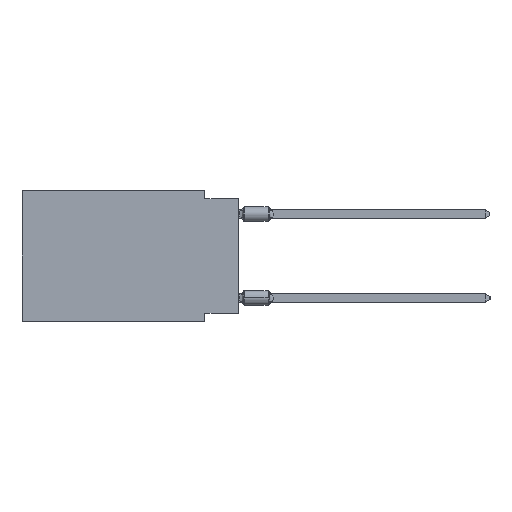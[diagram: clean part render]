
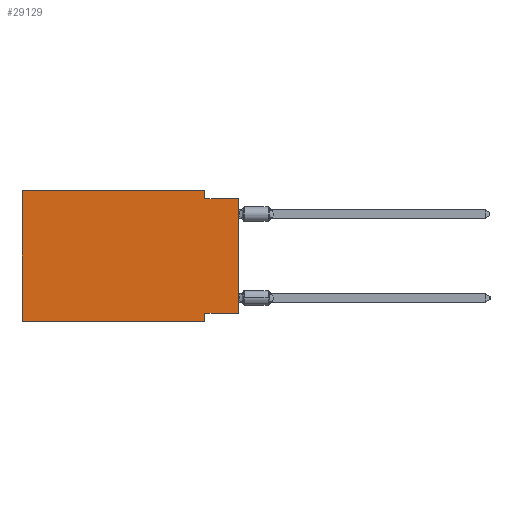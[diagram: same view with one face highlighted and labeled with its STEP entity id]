
A CAD part, left-side view. The second image highlights one B-rep face of the part: STEP entity #29129.
In plain terms, the highlighted planar face has unit normal (-1, 0, 0).
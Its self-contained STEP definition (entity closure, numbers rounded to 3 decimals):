
#415 = CARTESIAN_POINT ( 'NONE',  ( 0., 0., -0.635 ) ) ;
#2485 = DIRECTION ( 'NONE',  ( 0., 0., 1. ) ) ;
#3029 = VECTOR ( 'NONE', #5232, 1000. ) ;
#4148 = CARTESIAN_POINT ( 'NONE',  ( 0., 2.54, -9.271 ) ) ;
#4534 = VERTEX_POINT ( 'NONE', #4148 ) ;
#4603 = CARTESIAN_POINT ( 'NONE',  ( 0., 2.54, -9.906 ) ) ;
#4970 = CARTESIAN_POINT ( 'NONE',  ( 0., 0., 0. ) ) ;
#5232 = DIRECTION ( 'NONE',  ( 0., 0., -1. ) ) ;
#5471 = DIRECTION ( 'NONE',  ( 0., -1., 0. ) ) ;
#5879 = CARTESIAN_POINT ( 'NONE',  ( 0., 16.383, -9.906 ) ) ;
#6589 = EDGE_CURVE ( 'NONE', #14756, #17902, #17943, .T. ) ;
#6800 = DIRECTION ( 'NONE',  ( 0., 0., -1. ) ) ;
#8611 = LINE ( 'NONE', #23446, #3029 ) ;
#8615 = ORIENTED_EDGE ( 'NONE', *, *, #6589, .F. ) ;
#8883 = CARTESIAN_POINT ( 'NONE',  ( 0., 16.383, 0. ) ) ;
#9134 = VECTOR ( 'NONE', #5471, 1000. ) ;
#9616 = CARTESIAN_POINT ( 'NONE',  ( 0., 16.383, -9.906 ) ) ;
#9969 = CARTESIAN_POINT ( 'NONE',  ( 0., 16.383, 0. ) ) ;
#10181 = CARTESIAN_POINT ( 'NONE',  ( 0., 0., -9.271 ) ) ;
#10242 = EDGE_CURVE ( 'NONE', #4534, #38277, #22647, .T. ) ;
#12531 = AXIS2_PLACEMENT_3D ( 'NONE', #34232, #12992, #6800 ) ;
#12992 = DIRECTION ( 'NONE',  ( 1., 0., 0. ) ) ;
#13170 = EDGE_LOOP ( 'NONE', ( #30007, #8615, #27087, #38265, #25203, #16154, #23225, #16881 ) ) ;
#13526 = VERTEX_POINT ( 'NONE', #9616 ) ;
#14756 = VERTEX_POINT ( 'NONE', #33330 ) ;
#15594 = DIRECTION ( 'NONE',  ( 0., 1., 0. ) ) ;
#16154 = ORIENTED_EDGE ( 'NONE', *, *, #23469, .T. ) ;
#16581 = VECTOR ( 'NONE', #33555, 1000. ) ;
#16881 = ORIENTED_EDGE ( 'NONE', *, *, #32863, .F. ) ;
#17902 = VERTEX_POINT ( 'NONE', #415 ) ;
#17943 = LINE ( 'NONE', #20752, #16581 ) ;
#18418 = LINE ( 'NONE', #10181, #37679 ) ;
#18571 = CARTESIAN_POINT ( 'NONE',  ( 0., 2.54, 0. ) ) ;
#20137 = VERTEX_POINT ( 'NONE', #34807 ) ;
#20752 = CARTESIAN_POINT ( 'NONE',  ( 0., 0., -0.635 ) ) ;
#21342 = VERTEX_POINT ( 'NONE', #23188 ) ;
#21418 = CARTESIAN_POINT ( 'NONE',  ( 0., 2.54, -9.906 ) ) ;
#21791 = VECTOR ( 'NONE', #23009, 1000. ) ;
#22647 = LINE ( 'NONE', #4603, #37305 ) ;
#23009 = DIRECTION ( 'NONE',  ( 0., 0., 1. ) ) ;
#23188 = CARTESIAN_POINT ( 'NONE',  ( 0., 16.383, 0. ) ) ;
#23225 = ORIENTED_EDGE ( 'NONE', *, *, #10242, .F. ) ;
#23233 = DIRECTION ( 'NONE',  ( 0., 0., -1. ) ) ;
#23446 = CARTESIAN_POINT ( 'NONE',  ( 0., 2.54, 0. ) ) ;
#23469 = EDGE_CURVE ( 'NONE', #13526, #38277, #38944, .T. ) ;
#24162 = VECTOR ( 'NONE', #34425, 1000. ) ;
#24653 = EDGE_CURVE ( 'NONE', #13526, #21342, #29913, .T. ) ;
#25203 = ORIENTED_EDGE ( 'NONE', *, *, #24653, .F. ) ;
#25213 = LINE ( 'NONE', #9969, #24162 ) ;
#27087 = ORIENTED_EDGE ( 'NONE', *, *, #28869, .F. ) ;
#28238 = PLANE ( 'NONE',  #12531 ) ;
#28631 = FACE_OUTER_BOUND ( 'NONE', #13170, .T. ) ;
#28869 = EDGE_CURVE ( 'NONE', #33150, #14756, #8611, .T. ) ;
#29129 = ADVANCED_FACE ( 'NONE', ( #28631 ), #28238, .F. ) ;
#29738 = VECTOR ( 'NONE', #2485, 1000. ) ;
#29913 = LINE ( 'NONE', #8883, #29738 ) ;
#30007 = ORIENTED_EDGE ( 'NONE', *, *, #34745, .T. ) ;
#31595 = EDGE_CURVE ( 'NONE', #21342, #33150, #25213, .T. ) ;
#32863 = EDGE_CURVE ( 'NONE', #20137, #4534, #18418, .T. ) ;
#33150 = VERTEX_POINT ( 'NONE', #18571 ) ;
#33330 = CARTESIAN_POINT ( 'NONE',  ( 0., 2.54, -0.635 ) ) ;
#33555 = DIRECTION ( 'NONE',  ( 0., -1., 0. ) ) ;
#34232 = CARTESIAN_POINT ( 'NONE',  ( 0., 16.383, 0. ) ) ;
#34425 = DIRECTION ( 'NONE',  ( 0., -1., 0. ) ) ;
#34745 = EDGE_CURVE ( 'NONE', #20137, #17902, #38234, .T. ) ;
#34807 = CARTESIAN_POINT ( 'NONE',  ( 0., 0., -9.271 ) ) ;
#37305 = VECTOR ( 'NONE', #23233, 1000. ) ;
#37679 = VECTOR ( 'NONE', #15594, 1000. ) ;
#38234 = LINE ( 'NONE', #4970, #21791 ) ;
#38265 = ORIENTED_EDGE ( 'NONE', *, *, #31595, .F. ) ;
#38277 = VERTEX_POINT ( 'NONE', #21418 ) ;
#38944 = LINE ( 'NONE', #5879, #9134 ) ;
